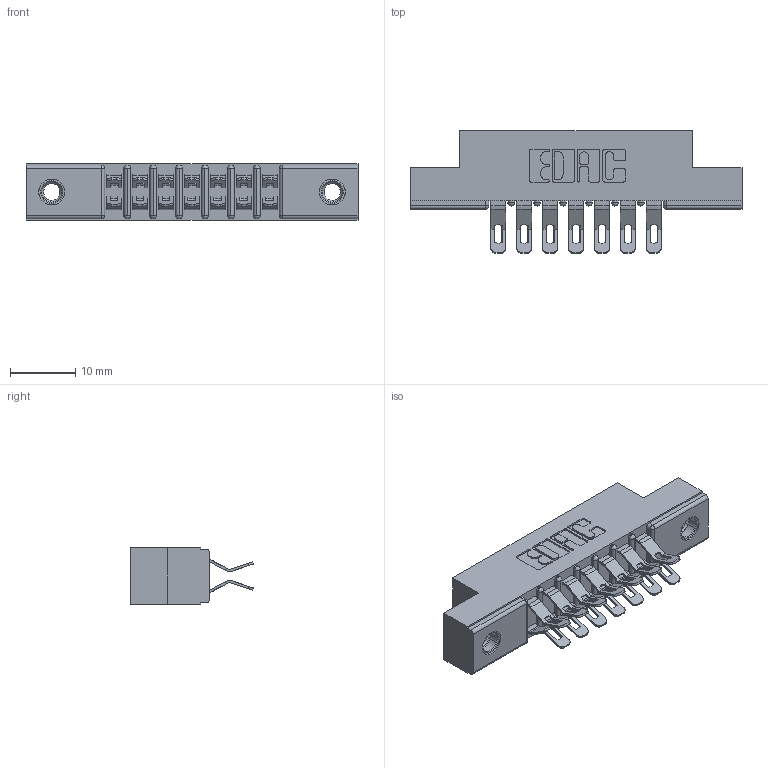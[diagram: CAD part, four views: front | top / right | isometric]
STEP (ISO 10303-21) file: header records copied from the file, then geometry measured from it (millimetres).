
FILE_DESCRIPTION (( 'STEP AP203' ), '1' );
FILE_NAME ('357-014-455-207.STEP', '2020-10-02T18:00:28', ( '' ), ( '' ), 'SwSTEP 2.0', 'SolidWorks 2020', '' );
FILE_SCHEMA (( 'CONFIG_CONTROL_DESIGN' ));
Length unit declared in the file: inch
Products named in the file (4): 345-250-001_345-250-005-103; 307 Part_.156 Dia Mounting Holes; 307-290-001_555; 357-014-455-207
Assembly tree (17 placements, depth 2):
  357-014-455-207
    307 Part_.156 Dia Mounting Holes
    307-290-001_555  x14
    345-250-001_345-250-005-103  x2
Bounding box: 50.75 x 18.75 x 8.71 mm (x, y, z)
Volume: 3349.4 mm3; surface area: 5402.2 mm2
Topology: 17 solids, 17 shells, 1040 faces, 2993 edges, 1946 vertices
Faces by surface type: plane 578, cylinder 430, sphere 16, cone 12, torus 4
Entity records: 12262 total; most frequent: CARTESIAN_POINT 2006, DIRECTION 1996, ORIENTED_EDGE 1980, EDGE_CURVE 990, VECTOR 732, LINE 732, VERTEX_POINT 642, AXIS2_PLACEMENT_3D 632
